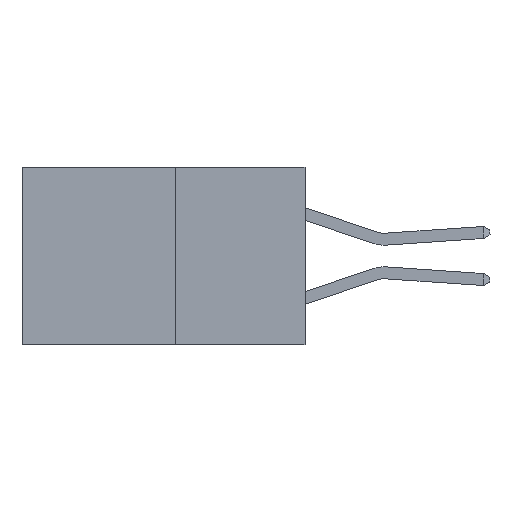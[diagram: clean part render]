
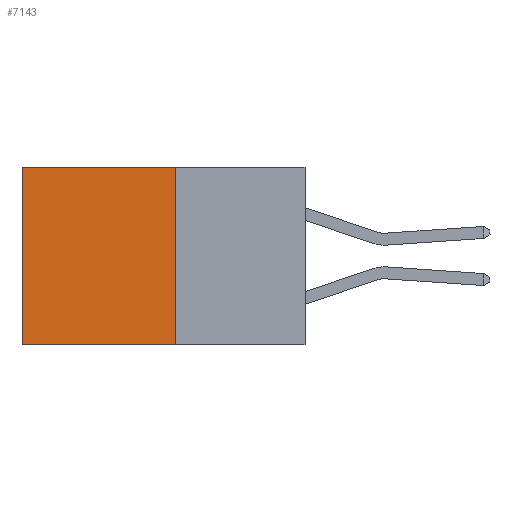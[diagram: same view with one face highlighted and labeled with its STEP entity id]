
A CAD part, left-side view. The second image highlights one B-rep face of the part: STEP entity #7143.
In plain terms, the highlighted planar face has unit normal (-1, 0, 0).
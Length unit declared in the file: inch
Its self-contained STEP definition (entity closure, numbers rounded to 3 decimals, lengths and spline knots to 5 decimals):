
#389 = VERTEX_POINT ( 'NONE', #2809 ) ;
#419 = VECTOR ( 'NONE', #9101, 39.37008 ) ;
#1115 = PLANE ( 'NONE',  #8585 ) ;
#2068 = DIRECTION ( 'NONE',  ( 1., 0., 0. ) ) ;
#2405 = CARTESIAN_POINT ( 'NONE',  ( 0.277, 0.27, -0.37 ) ) ;
#2775 = DIRECTION ( 'NONE',  ( 0., 1., 0. ) ) ;
#2809 = CARTESIAN_POINT ( 'NONE',  ( 0.277, 0.59, 0. ) ) ;
#3034 = VECTOR ( 'NONE', #6567, 39.37008 ) ;
#3204 = ORIENTED_EDGE ( 'NONE', *, *, #5481, .F. ) ;
#4088 = CARTESIAN_POINT ( 'NONE',  ( 0.277, 0.59, -0.37 ) ) ;
#4350 = CARTESIAN_POINT ( 'NONE',  ( 0.277, 0.59, -0.37 ) ) ;
#4872 = EDGE_CURVE ( 'NONE', #389, #9783, #11714, .T. ) ;
#5220 = VERTEX_POINT ( 'NONE', #9685 ) ;
#5481 = EDGE_CURVE ( 'NONE', #5220, #12091, #5743, .T. ) ;
#5626 = CARTESIAN_POINT ( 'NONE',  ( 0.277, 0.27, 0. ) ) ;
#5743 = LINE ( 'NONE', #2405, #419 ) ;
#6567 = DIRECTION ( 'NONE',  ( 0., 1., 0. ) ) ;
#7143 = ADVANCED_FACE ( 'NONE', ( #12205 ), #1115, .F. ) ;
#7509 = CARTESIAN_POINT ( 'NONE',  ( 0.277, 0.27, -0.37 ) ) ;
#7787 = CARTESIAN_POINT ( 'NONE',  ( 0.277, 0.27, -0.37 ) ) ;
#8096 = LINE ( 'NONE', #5626, #3034 ) ;
#8585 = AXIS2_PLACEMENT_3D ( 'NONE', #7787, #2068, #8779 ) ;
#8779 = DIRECTION ( 'NONE',  ( 0., 0., -1. ) ) ;
#8943 = EDGE_CURVE ( 'NONE', #5220, #389, #8096, .T. ) ;
#8985 = EDGE_LOOP ( 'NONE', ( #9603, #12028, #3204, #11939 ) ) ;
#9101 = DIRECTION ( 'NONE',  ( 0., 0., -1. ) ) ;
#9531 = VECTOR ( 'NONE', #2775, 39.37008 ) ;
#9603 = ORIENTED_EDGE ( 'NONE', *, *, #4872, .T. ) ;
#9685 = CARTESIAN_POINT ( 'NONE',  ( 0.277, 0.27, 0. ) ) ;
#9695 = CARTESIAN_POINT ( 'NONE',  ( 0.277, 0.27, -0.37 ) ) ;
#9783 = VERTEX_POINT ( 'NONE', #4088 ) ;
#10999 = DIRECTION ( 'NONE',  ( 0., 0., -1. ) ) ;
#11714 = LINE ( 'NONE', #4350, #11983 ) ;
#11916 = EDGE_CURVE ( 'NONE', #12091, #9783, #11980, .T. ) ;
#11939 = ORIENTED_EDGE ( 'NONE', *, *, #8943, .T. ) ;
#11980 = LINE ( 'NONE', #7509, #9531 ) ;
#11983 = VECTOR ( 'NONE', #10999, 39.37008 ) ;
#12028 = ORIENTED_EDGE ( 'NONE', *, *, #11916, .F. ) ;
#12091 = VERTEX_POINT ( 'NONE', #9695 ) ;
#12205 = FACE_OUTER_BOUND ( 'NONE', #8985, .T. ) ;
